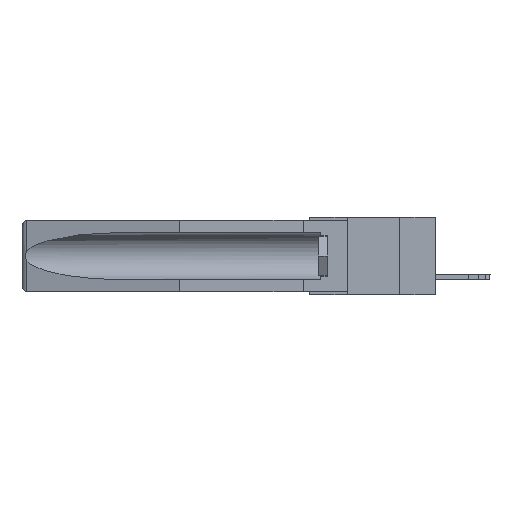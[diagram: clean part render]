
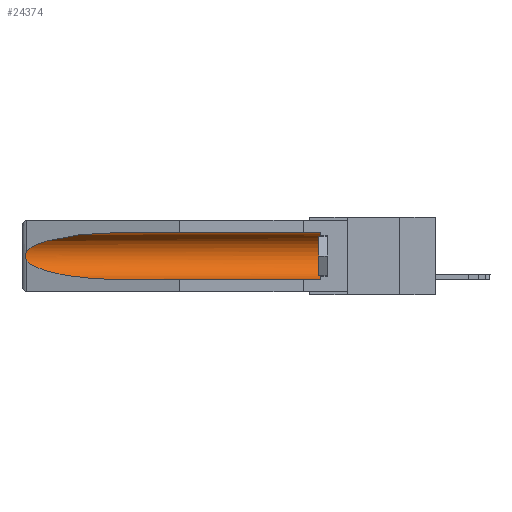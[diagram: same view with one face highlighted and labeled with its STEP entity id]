
A CAD part, left-side view. The second image highlights one B-rep face of the part: STEP entity #24374.
In plain terms, the highlighted cylindrical face has radius 2.857 mm (diameter 5.715 mm), a partial arc.
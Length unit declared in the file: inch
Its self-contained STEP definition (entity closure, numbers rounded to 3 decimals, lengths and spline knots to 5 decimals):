
#787 = CARTESIAN_POINT ( 'NONE',  ( 0.26654, 1.53092, -0.15636 ) ) ;
#1694 = LINE ( 'NONE', #20444, #20530 ) ;
#1726 = CARTESIAN_POINT ( 'NONE',  ( 0.26537, 1.52718, -0.19328 ) ) ;
#3272 = ORIENTED_EDGE ( 'NONE', *, *, #20035, .T. ) ;
#3287 = EDGE_LOOP ( 'NONE', ( #3623, #3272, #24882, #4172, #9711, #20951 ) ) ;
#3381 =( BOUNDED_CURVE ( )  B_SPLINE_CURVE ( 3, ( #5767, #20232, #11901, #22270 ),
 .UNSPECIFIED., .F., .F. ) 
 B_SPLINE_CURVE_WITH_KNOTS ( ( 4, 4 ),
 ( 4.71239, 6.08839 ),
 .UNSPECIFIED. ) 
 CURVE ( )  GEOMETRIC_REPRESENTATION_ITEM ( )  RATIONAL_B_SPLINE_CURVE ( ( 1., 0.848, 0.848, 1. ) ) 
 REPRESENTATION_ITEM ( '' )  );
#3623 = ORIENTED_EDGE ( 'NONE', *, *, #19227, .T. ) ;
#4172 = ORIENTED_EDGE ( 'NONE', *, *, #19376, .F. ) ;
#4321 = DIRECTION ( 'NONE',  ( 0., 1., 0. ) ) ;
#4773 = CARTESIAN_POINT ( 'NONE',  ( 0.2673, 1.5327, -0.16383 ) ) ;
#4857 = CARTESIAN_POINT ( 'NONE',  ( 0.26537, 1.52718, -0.19328 ) ) ;
#5074 = LINE ( 'NONE', #11001, #24573 ) ;
#5767 = CARTESIAN_POINT ( 'NONE',  ( 0.155, 1.07973, -0.059 ) ) ;
#6161 = EDGE_CURVE ( 'NONE', #14468, #6466, #25391, .T. ) ;
#6466 = VERTEX_POINT ( 'NONE', #10581 ) ;
#6681 = EDGE_CURVE ( 'NONE', #9451, #17935, #21601, .T. ) ;
#6767 = DIRECTION ( 'NONE',  ( 0., 1., 0. ) ) ;
#7677 = VERTEX_POINT ( 'NONE', #9370 ) ;
#9370 = CARTESIAN_POINT ( 'NONE',  ( 0.155, 1.07973, -0.059 ) ) ;
#9411 = CARTESIAN_POINT ( 'NONE',  ( 0.26537, 1.52718, -0.14972 ) ) ;
#9451 = VERTEX_POINT ( 'NONE', #9528 ) ;
#9528 = CARTESIAN_POINT ( 'NONE',  ( 0.155, 0.126, -0.284 ) ) ;
#9581 = CARTESIAN_POINT ( 'NONE',  ( 0.155, 1.07973, -0.284 ) ) ;
#9711 = ORIENTED_EDGE ( 'NONE', *, *, #6681, .T. ) ;
#10008 = CARTESIAN_POINT ( 'NONE',  ( 0.155, -0.30754, -0.1715 ) ) ;
#10186 = DIRECTION ( 'NONE',  ( 0., 0., 1. ) ) ;
#10362 = EDGE_CURVE ( 'NONE', #17935, #7677, #1694, .T. ) ;
#10581 = CARTESIAN_POINT ( 'NONE',  ( 0.155, 1.07973, -0.284 ) ) ;
#10987 = CARTESIAN_POINT ( 'NONE',  ( 0.2673, 1.53269, -0.17917 ) ) ;
#11001 = CARTESIAN_POINT ( 'NONE',  ( 0.155, -0.30754, -0.284 ) ) ;
#11901 = CARTESIAN_POINT ( 'NONE',  ( 0.25451, 1.48313, -0.09465 ) ) ;
#12409 = DIRECTION ( 'NONE',  ( 0., -1., 0. ) ) ;
#13012 = CARTESIAN_POINT ( 'NONE',  ( 0.26655, 1.53094, -0.18657 ) ) ;
#13790 = CARTESIAN_POINT ( 'NONE',  ( 0.21114, 1.30732, -0.284 ) ) ;
#14092 = AXIS2_PLACEMENT_3D ( 'NONE', #18425, #12409, #16259 ) ;
#14468 = VERTEX_POINT ( 'NONE', #1726 ) ;
#14792 = B_SPLINE_CURVE_WITH_KNOTS ( 'NONE', 3,
 ( #24763, #18968, #787, #4773, #17069, #14920, #10987, #13012, #19053, #4857 ),
 .UNSPECIFIED., .F., .F.,
 ( 4, 2, 2, 2, 4 ),
 ( 0., 0.00029, 0.00058, 0.00087, 0.00117 ),
 .UNSPECIFIED. ) ;
#14920 = CARTESIAN_POINT ( 'NONE',  ( 0.2675, 1.53308, -0.17534 ) ) ;
#15762 = CARTESIAN_POINT ( 'NONE',  ( 0.25451, 1.48313, -0.24835 ) ) ;
#15892 = VERTEX_POINT ( 'NONE', #9411 ) ;
#16259 = DIRECTION ( 'NONE',  ( 0., 0., 1. ) ) ;
#16261 = DIRECTION ( 'NONE',  ( 0., 1., 0. ) ) ;
#16597 = CYLINDRICAL_SURFACE ( 'NONE', #25300, 0.1125 ) ;
#17069 = CARTESIAN_POINT ( 'NONE',  ( 0.2675, 1.53308, -0.16763 ) ) ;
#17935 = VERTEX_POINT ( 'NONE', #22021 ) ;
#18425 = CARTESIAN_POINT ( 'NONE',  ( 0.155, 0.126, -0.1715 ) ) ;
#18968 = CARTESIAN_POINT ( 'NONE',  ( 0.26597, 1.52961, -0.15275 ) ) ;
#19053 = CARTESIAN_POINT ( 'NONE',  ( 0.26597, 1.5296, -0.19026 ) ) ;
#19227 = EDGE_CURVE ( 'NONE', #7677, #15892, #3381, .T. ) ;
#19376 = EDGE_CURVE ( 'NONE', #9451, #6466, #5074, .T. ) ;
#19807 = FACE_OUTER_BOUND ( 'NONE', #3287, .T. ) ;
#20035 = EDGE_CURVE ( 'NONE', #15892, #14468, #14792, .T. ) ;
#20071 = CARTESIAN_POINT ( 'NONE',  ( 0.26537, 1.52718, -0.19328 ) ) ;
#20232 = CARTESIAN_POINT ( 'NONE',  ( 0.21114, 1.30732, -0.059 ) ) ;
#20444 = CARTESIAN_POINT ( 'NONE',  ( 0.155, -0.30754, -0.059 ) ) ;
#20530 = VECTOR ( 'NONE', #4321, 39.37008 ) ;
#20951 = ORIENTED_EDGE ( 'NONE', *, *, #10362, .T. ) ;
#21601 = CIRCLE ( 'NONE', #14092, 0.1125 ) ;
#22021 = CARTESIAN_POINT ( 'NONE',  ( 0.155, 0.126, -0.059 ) ) ;
#22270 = CARTESIAN_POINT ( 'NONE',  ( 0.26537, 1.52718, -0.14972 ) ) ;
#24374 = ADVANCED_FACE ( 'NONE', ( #19807 ), #16597, .F. ) ;
#24573 = VECTOR ( 'NONE', #6767, 39.37008 ) ;
#24763 = CARTESIAN_POINT ( 'NONE',  ( 0.26537, 1.52718, -0.14972 ) ) ;
#24882 = ORIENTED_EDGE ( 'NONE', *, *, #6161, .T. ) ;
#25300 = AXIS2_PLACEMENT_3D ( 'NONE', #10008, #16261, #10186 ) ;
#25391 =( BOUNDED_CURVE ( )  B_SPLINE_CURVE ( 3, ( #20071, #15762, #13790, #9581 ),
 .UNSPECIFIED., .F., .F. ) 
 B_SPLINE_CURVE_WITH_KNOTS ( ( 4, 4 ),
 ( 0.1948, 1.5708 ),
 .UNSPECIFIED. ) 
 CURVE ( )  GEOMETRIC_REPRESENTATION_ITEM ( )  RATIONAL_B_SPLINE_CURVE ( ( 1., 0.848, 0.848, 1. ) ) 
 REPRESENTATION_ITEM ( '' )  );
